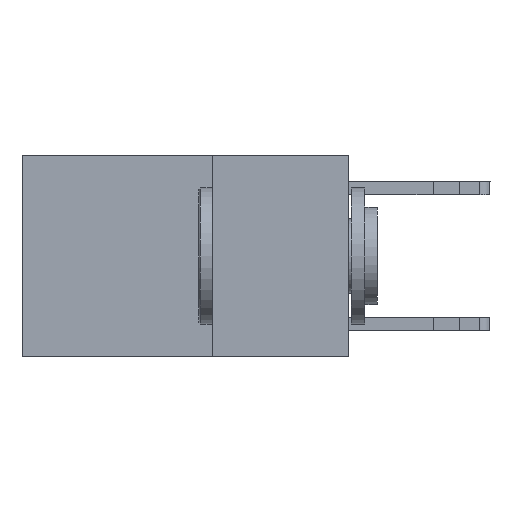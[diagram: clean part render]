
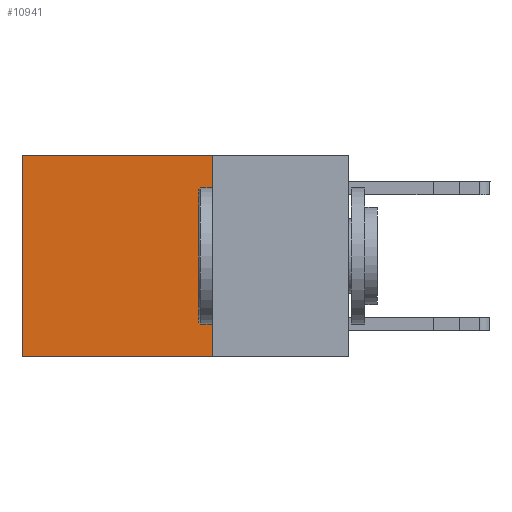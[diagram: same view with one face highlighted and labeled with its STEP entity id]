
A CAD part, left-side view. The second image highlights one B-rep face of the part: STEP entity #10941.
In plain terms, the highlighted planar face has unit normal (-1, 0, 0).
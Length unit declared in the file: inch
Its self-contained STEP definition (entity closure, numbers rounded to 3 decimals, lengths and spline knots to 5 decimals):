
#522 = CARTESIAN_POINT ( 'NONE',  ( 0.2625, 0.25, 0. ) ) ;
#649 = DIRECTION ( 'NONE',  ( 1., 0., 0. ) ) ;
#863 = ORIENTED_EDGE ( 'NONE', *, *, #5736, .T. ) ;
#1672 = CARTESIAN_POINT ( 'NONE',  ( 0.2625, 0.6, -0.37 ) ) ;
#1684 = EDGE_CURVE ( 'NONE', #3985, #19119, #1712, .T. ) ;
#1712 = LINE ( 'NONE', #20681, #5447 ) ;
#2114 = LINE ( 'NONE', #16955, #14872 ) ;
#3828 = DIRECTION ( 'NONE',  ( 0., 1., 0. ) ) ;
#3932 = ORIENTED_EDGE ( 'NONE', *, *, #20397, .T. ) ;
#3985 = VERTEX_POINT ( 'NONE', #9031 ) ;
#4553 = FACE_OUTER_BOUND ( 'NONE', #10277, .T. ) ;
#5026 = CARTESIAN_POINT ( 'NONE',  ( 0.2625, 0.6, 0. ) ) ;
#5144 = DIRECTION ( 'NONE',  ( 0., 1., 0. ) ) ;
#5447 = VECTOR ( 'NONE', #3828, 39.37008 ) ;
#5736 = EDGE_CURVE ( 'NONE', #15377, #11075, #16217, .T. ) ;
#6794 = LINE ( 'NONE', #5026, #21387 ) ;
#7878 = DIRECTION ( 'NONE',  ( 0., 0., -1. ) ) ;
#8188 = DIRECTION ( 'NONE',  ( 0., 0., -1. ) ) ;
#8918 = CARTESIAN_POINT ( 'NONE',  ( 0.2625, 0.25, 0. ) ) ;
#9031 = CARTESIAN_POINT ( 'NONE',  ( 0.2625, 0.25, -0.37 ) ) ;
#9433 = AXIS2_PLACEMENT_3D ( 'NONE', #522, #649, #8188 ) ;
#10277 = EDGE_LOOP ( 'NONE', ( #3932, #14941, #18287, #863 ) ) ;
#10941 = ADVANCED_FACE ( 'NONE', ( #4553 ), #17744, .F. ) ;
#11075 = VERTEX_POINT ( 'NONE', #16739 ) ;
#12465 = VECTOR ( 'NONE', #5144, 39.37008 ) ;
#12837 = DIRECTION ( 'NONE',  ( 0., 0., -1. ) ) ;
#14872 = VECTOR ( 'NONE', #7878, 39.37008 ) ;
#14941 = ORIENTED_EDGE ( 'NONE', *, *, #1684, .F. ) ;
#15377 = VERTEX_POINT ( 'NONE', #8918 ) ;
#16217 = LINE ( 'NONE', #16585, #12465 ) ;
#16365 = EDGE_CURVE ( 'NONE', #15377, #3985, #2114, .T. ) ;
#16585 = CARTESIAN_POINT ( 'NONE',  ( 0.2625, 0.25, 0. ) ) ;
#16739 = CARTESIAN_POINT ( 'NONE',  ( 0.2625, 0.6, 0. ) ) ;
#16955 = CARTESIAN_POINT ( 'NONE',  ( 0.2625, 0.25, 0. ) ) ;
#17744 = PLANE ( 'NONE',  #9433 ) ;
#18287 = ORIENTED_EDGE ( 'NONE', *, *, #16365, .F. ) ;
#19119 = VERTEX_POINT ( 'NONE', #1672 ) ;
#20397 = EDGE_CURVE ( 'NONE', #11075, #19119, #6794, .T. ) ;
#20681 = CARTESIAN_POINT ( 'NONE',  ( 0.2625, 0.25, -0.37 ) ) ;
#21387 = VECTOR ( 'NONE', #12837, 39.37008 ) ;
